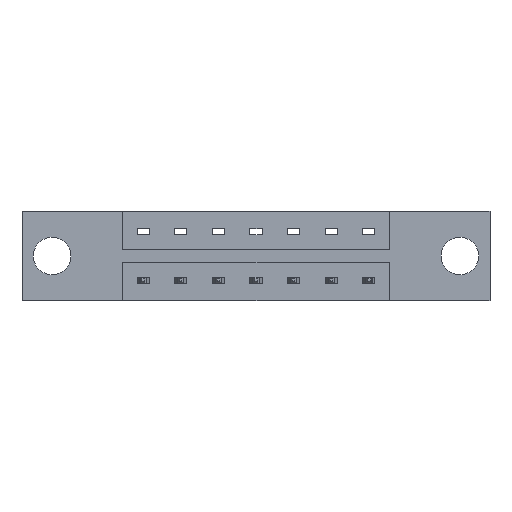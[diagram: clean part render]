
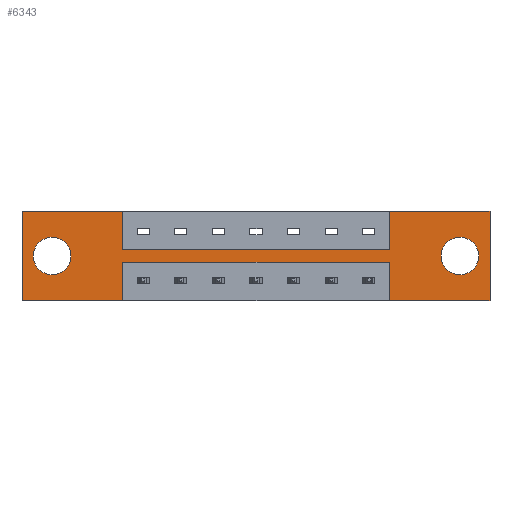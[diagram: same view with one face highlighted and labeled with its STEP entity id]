
A CAD part, front view. The second image highlights one B-rep face of the part: STEP entity #6343.
In plain terms, the highlighted planar face has unit normal (0, -1, 0).
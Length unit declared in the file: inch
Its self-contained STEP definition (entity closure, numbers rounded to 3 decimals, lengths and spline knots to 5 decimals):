
#145 = CARTESIAN_POINT ( 'NONE',  ( 1.815, 0., -0.185 ) ) ;
#204 = AXIS2_PLACEMENT_3D ( 'NONE', #1064, #2256, #6292 ) ;
#210 = CARTESIAN_POINT ( 'NONE',  ( 0., 0., -0.37 ) ) ;
#308 = DIRECTION ( 'NONE',  ( 0., -1., 0. ) ) ;
#342 = EDGE_LOOP ( 'NONE', ( #3993, #2264, #3940, #5503, #2034, #6940, #2695, #8506, #3206, #5954, #5889, #2539 ) ) ;
#528 = DIRECTION ( 'NONE',  ( 0., 0., -1. ) ) ;
#571 = EDGE_CURVE ( 'NONE', #3131, #4682, #7152, .T. ) ;
#756 = LINE ( 'NONE', #3507, #1059 ) ;
#844 = DIRECTION ( 'NONE',  ( 0., 0., 1. ) ) ;
#858 = CARTESIAN_POINT ( 'NONE',  ( 0.4175, 0., 0. ) ) ;
#888 = CIRCLE ( 'NONE', #5898, 0.078 ) ;
#934 = AXIS2_PLACEMENT_3D ( 'NONE', #145, #7670, #2362 ) ;
#939 = PLANE ( 'NONE',  #2218 ) ;
#1004 = EDGE_CURVE ( 'NONE', #4912, #3233, #2453, .T. ) ;
#1059 = VECTOR ( 'NONE', #3581, 39.37008 ) ;
#1064 = CARTESIAN_POINT ( 'NONE',  ( 0.125, 0., -0.185 ) ) ;
#1122 = EDGE_CURVE ( 'NONE', #5126, #4912, #4687, .T. ) ;
#1329 = LINE ( 'NONE', #6790, #7149 ) ;
#1362 = CARTESIAN_POINT ( 'NONE',  ( 1.94, 0., -0.37 ) ) ;
#1372 = CARTESIAN_POINT ( 'NONE',  ( 1.5225, 0., -0.37 ) ) ;
#1374 = VERTEX_POINT ( 'NONE', #8590 ) ;
#1397 = CARTESIAN_POINT ( 'NONE',  ( 1.94, 0., 0. ) ) ;
#1616 = CARTESIAN_POINT ( 'NONE',  ( 1.5225, 0., 0. ) ) ;
#1619 = EDGE_CURVE ( 'NONE', #4682, #1374, #5197, .T. ) ;
#1630 = EDGE_CURVE ( 'NONE', #3867, #4654, #888, .T. ) ;
#1691 = CARTESIAN_POINT ( 'NONE',  ( 0.4175, 0., -0.2115 ) ) ;
#1694 = DIRECTION ( 'NONE',  ( 0., 0., 1. ) ) ;
#1704 = CARTESIAN_POINT ( 'NONE',  ( 0., 0., -0.37 ) ) ;
#1758 = LINE ( 'NONE', #5102, #5041 ) ;
#2034 = ORIENTED_EDGE ( 'NONE', *, *, #5476, .F. ) ;
#2076 = CARTESIAN_POINT ( 'NONE',  ( 1.5225, 0., -0.2115 ) ) ;
#2145 = EDGE_CURVE ( 'NONE', #5055, #3131, #1758, .T. ) ;
#2167 = EDGE_CURVE ( 'NONE', #5729, #2891, #4469, .T. ) ;
#2213 = VERTEX_POINT ( 'NONE', #2346 ) ;
#2218 = AXIS2_PLACEMENT_3D ( 'NONE', #6307, #308, #3558 ) ;
#2256 = DIRECTION ( 'NONE',  ( 0., 1., 0. ) ) ;
#2264 = ORIENTED_EDGE ( 'NONE', *, *, #7527, .F. ) ;
#2293 = CARTESIAN_POINT ( 'NONE',  ( 0.125, 0., -0.185 ) ) ;
#2302 = FACE_OUTER_BOUND ( 'NONE', #342, .T. ) ;
#2346 = CARTESIAN_POINT ( 'NONE',  ( 1.5225, 0., -0.1585 ) ) ;
#2362 = DIRECTION ( 'NONE',  ( 0., 0., -1. ) ) ;
#2414 = DIRECTION ( 'NONE',  ( 0., 0., -1. ) ) ;
#2453 = LINE ( 'NONE', #7896, #3900 ) ;
#2474 = CARTESIAN_POINT ( 'NONE',  ( 1.815, 0., -0.185 ) ) ;
#2539 = ORIENTED_EDGE ( 'NONE', *, *, #3672, .F. ) ;
#2695 = ORIENTED_EDGE ( 'NONE', *, *, #1619, .F. ) ;
#2891 = VERTEX_POINT ( 'NONE', #2076 ) ;
#3007 = CARTESIAN_POINT ( 'NONE',  ( 0.4175, 0., -0.1585 ) ) ;
#3013 = VECTOR ( 'NONE', #528, 39.37008 ) ;
#3055 = CARTESIAN_POINT ( 'NONE',  ( 0., 0., 0. ) ) ;
#3084 = VECTOR ( 'NONE', #7857, 39.37008 ) ;
#3131 = VERTEX_POINT ( 'NONE', #8115 ) ;
#3206 = ORIENTED_EDGE ( 'NONE', *, *, #2145, .F. ) ;
#3224 = ORIENTED_EDGE ( 'NONE', *, *, #3806, .T. ) ;
#3233 = VERTEX_POINT ( 'NONE', #1362 ) ;
#3456 = AXIS2_PLACEMENT_3D ( 'NONE', #2293, #4887, #8320 ) ;
#3507 = CARTESIAN_POINT ( 'NONE',  ( 0.4175, 0., -0.2115 ) ) ;
#3558 = DIRECTION ( 'NONE',  ( 0., 0., -1. ) ) ;
#3581 = DIRECTION ( 'NONE',  ( -1., 0., 0. ) ) ;
#3616 = CARTESIAN_POINT ( 'NONE',  ( 1.5225, 0., -0.1585 ) ) ;
#3658 = CIRCLE ( 'NONE', #934, 0.078 ) ;
#3672 = EDGE_CURVE ( 'NONE', #2891, #4252, #756, .T. ) ;
#3712 = EDGE_CURVE ( 'NONE', #4630, #5055, #8517, .T. ) ;
#3766 = CARTESIAN_POINT ( 'NONE',  ( 1.5225, 0., -0.2115 ) ) ;
#3806 = EDGE_CURVE ( 'NONE', #7812, #8318, #7779, .T. ) ;
#3867 = VERTEX_POINT ( 'NONE', #5989 ) ;
#3894 = ORIENTED_EDGE ( 'NONE', *, *, #1630, .T. ) ;
#3900 = VECTOR ( 'NONE', #2414, 39.37008 ) ;
#3940 = ORIENTED_EDGE ( 'NONE', *, *, #1004, .F. ) ;
#3993 = ORIENTED_EDGE ( 'NONE', *, *, #2167, .F. ) ;
#4155 = EDGE_CURVE ( 'NONE', #1374, #2213, #8343, .T. ) ;
#4252 = VERTEX_POINT ( 'NONE', #1691 ) ;
#4311 = VECTOR ( 'NONE', #5979, 39.37008 ) ;
#4469 = LINE ( 'NONE', #3766, #7895 ) ;
#4630 = VERTEX_POINT ( 'NONE', #7087 ) ;
#4654 = VERTEX_POINT ( 'NONE', #8404 ) ;
#4663 = CARTESIAN_POINT ( 'NONE',  ( 0.125, 0., -0.263 ) ) ;
#4682 = VERTEX_POINT ( 'NONE', #858 ) ;
#4687 = LINE ( 'NONE', #5936, #4311 ) ;
#4887 = DIRECTION ( 'NONE',  ( 0., 1., 0. ) ) ;
#4912 = VERTEX_POINT ( 'NONE', #1397 ) ;
#5041 = VECTOR ( 'NONE', #7823, 39.37008 ) ;
#5055 = VERTEX_POINT ( 'NONE', #1704 ) ;
#5102 = CARTESIAN_POINT ( 'NONE',  ( 0., 0., 0. ) ) ;
#5126 = VERTEX_POINT ( 'NONE', #1616 ) ;
#5197 = LINE ( 'NONE', #3007, #8592 ) ;
#5439 = DIRECTION ( 'NONE',  ( -1., 0., 0. ) ) ;
#5459 = VECTOR ( 'NONE', #7197, 39.37008 ) ;
#5476 = EDGE_CURVE ( 'NONE', #2213, #5126, #7807, .T. ) ;
#5503 = ORIENTED_EDGE ( 'NONE', *, *, #1122, .F. ) ;
#5695 = DIRECTION ( 'NONE',  ( 1., 0., 0. ) ) ;
#5729 = VERTEX_POINT ( 'NONE', #1372 ) ;
#5889 = ORIENTED_EDGE ( 'NONE', *, *, #7001, .F. ) ;
#5894 = EDGE_CURVE ( 'NONE', #4654, #3867, #3658, .T. ) ;
#5898 = AXIS2_PLACEMENT_3D ( 'NONE', #2474, #8523, #8567 ) ;
#5908 = DIRECTION ( 'NONE',  ( 0., 0., -1. ) ) ;
#5936 = CARTESIAN_POINT ( 'NONE',  ( 0., 0., 0. ) ) ;
#5954 = ORIENTED_EDGE ( 'NONE', *, *, #3712, .F. ) ;
#5979 = DIRECTION ( 'NONE',  ( 1., 0., 0. ) ) ;
#5989 = CARTESIAN_POINT ( 'NONE',  ( 1.815, 0., -0.263 ) ) ;
#6137 = CARTESIAN_POINT ( 'NONE',  ( 0.125, 0., -0.107 ) ) ;
#6292 = DIRECTION ( 'NONE',  ( 0., 0., 1. ) ) ;
#6307 = CARTESIAN_POINT ( 'NONE',  ( 0., 0., -0.37 ) ) ;
#6343 = ADVANCED_FACE ( 'NONE', ( #8445, #8398, #2302 ), #939, .T. ) ;
#6407 = CARTESIAN_POINT ( 'NONE',  ( 0.4175, 0., -0.1585 ) ) ;
#6572 = VECTOR ( 'NONE', #1694, 39.37008 ) ;
#6790 = CARTESIAN_POINT ( 'NONE',  ( 0., 0., -0.37 ) ) ;
#6833 = EDGE_LOOP ( 'NONE', ( #3224, #8707 ) ) ;
#6940 = ORIENTED_EDGE ( 'NONE', *, *, #4155, .F. ) ;
#7001 = EDGE_CURVE ( 'NONE', #4252, #4630, #8188, .T. ) ;
#7087 = CARTESIAN_POINT ( 'NONE',  ( 0.4175, 0., -0.37 ) ) ;
#7149 = VECTOR ( 'NONE', #5439, 39.37008 ) ;
#7152 = LINE ( 'NONE', #3055, #5459 ) ;
#7197 = DIRECTION ( 'NONE',  ( 1., 0., 0. ) ) ;
#7434 = EDGE_LOOP ( 'NONE', ( #7835, #3894 ) ) ;
#7507 = VECTOR ( 'NONE', #5695, 39.37008 ) ;
#7515 = CARTESIAN_POINT ( 'NONE',  ( 0.4175, 0., -0.2115 ) ) ;
#7527 = EDGE_CURVE ( 'NONE', #3233, #5729, #1329, .T. ) ;
#7670 = DIRECTION ( 'NONE',  ( 0., 1., 0. ) ) ;
#7779 = CIRCLE ( 'NONE', #204, 0.078 ) ;
#7807 = LINE ( 'NONE', #3616, #6572 ) ;
#7812 = VERTEX_POINT ( 'NONE', #6137 ) ;
#7823 = DIRECTION ( 'NONE',  ( 0., 0., 1. ) ) ;
#7835 = ORIENTED_EDGE ( 'NONE', *, *, #5894, .T. ) ;
#7857 = DIRECTION ( 'NONE',  ( -1., 0., 0. ) ) ;
#7866 = CIRCLE ( 'NONE', #3456, 0.078 ) ;
#7895 = VECTOR ( 'NONE', #844, 39.37008 ) ;
#7896 = CARTESIAN_POINT ( 'NONE',  ( 1.94, 0., 0. ) ) ;
#7994 = EDGE_CURVE ( 'NONE', #8318, #7812, #7866, .T. ) ;
#8115 = CARTESIAN_POINT ( 'NONE',  ( 0., 0., 0. ) ) ;
#8188 = LINE ( 'NONE', #7515, #3013 ) ;
#8318 = VERTEX_POINT ( 'NONE', #4663 ) ;
#8320 = DIRECTION ( 'NONE',  ( 0., 0., 1. ) ) ;
#8343 = LINE ( 'NONE', #6407, #7507 ) ;
#8398 = FACE_BOUND ( 'NONE', #6833, .T. ) ;
#8404 = CARTESIAN_POINT ( 'NONE',  ( 1.815, 0., -0.107 ) ) ;
#8445 = FACE_BOUND ( 'NONE', #7434, .T. ) ;
#8506 = ORIENTED_EDGE ( 'NONE', *, *, #571, .F. ) ;
#8517 = LINE ( 'NONE', #210, #3084 ) ;
#8523 = DIRECTION ( 'NONE',  ( 0., 1., 0. ) ) ;
#8567 = DIRECTION ( 'NONE',  ( 0., 0., -1. ) ) ;
#8590 = CARTESIAN_POINT ( 'NONE',  ( 0.4175, 0., -0.1585 ) ) ;
#8592 = VECTOR ( 'NONE', #5908, 39.37008 ) ;
#8707 = ORIENTED_EDGE ( 'NONE', *, *, #7994, .T. ) ;
